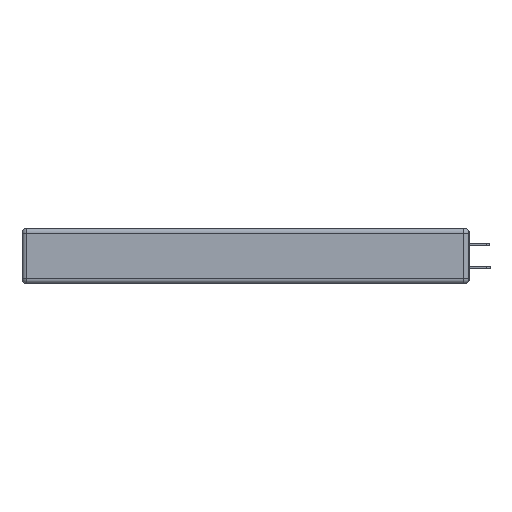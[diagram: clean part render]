
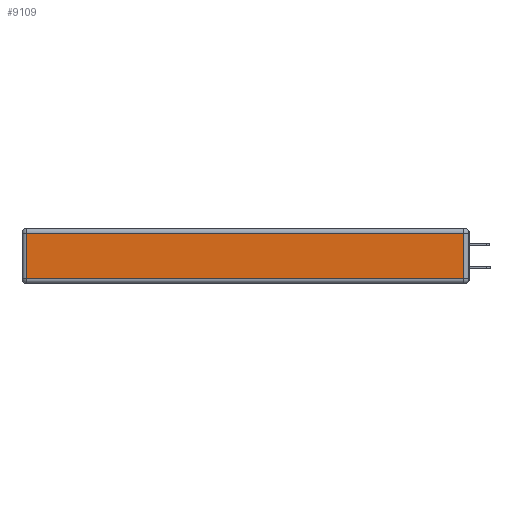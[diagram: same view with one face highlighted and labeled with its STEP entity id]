
A CAD part, left-side view. The second image highlights one B-rep face of the part: STEP entity #9109.
In plain terms, the highlighted planar face has unit normal (-1, 0, 0).
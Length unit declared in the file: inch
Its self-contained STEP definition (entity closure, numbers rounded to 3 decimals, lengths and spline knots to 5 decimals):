
#707 = EDGE_CURVE ( 'NONE', #20774, #18766, #6407, .T. ) ;
#1019 = DIRECTION ( 'NONE',  ( 0., 0., 1. ) ) ;
#1424 = DIRECTION ( 'NONE',  ( 0., 0., -1. ) ) ;
#2869 = EDGE_CURVE ( 'NONE', #13007, #16295, #25251, .T. ) ;
#2914 = VECTOR ( 'NONE', #23460, 39.37008 ) ;
#6209 = CARTESIAN_POINT ( 'NONE',  ( 0., 0.03, -0.03 ) ) ;
#6407 = LINE ( 'NONE', #9385, #2914 ) ;
#7319 = CARTESIAN_POINT ( 'NONE',  ( 0., 2.72, -0.03 ) ) ;
#8759 = CARTESIAN_POINT ( 'NONE',  ( 0., 0.03, -0.343 ) ) ;
#9070 = ORIENTED_EDGE ( 'NONE', *, *, #15851, .T. ) ;
#9109 = ADVANCED_FACE ( 'NONE', ( #24880 ), #24212, .T. ) ;
#9360 = VECTOR ( 'NONE', #1019, 39.37008 ) ;
#9385 = CARTESIAN_POINT ( 'NONE',  ( 0., 0., -0.313 ) ) ;
#9700 = LINE ( 'NONE', #8759, #9360 ) ;
#10495 = DIRECTION ( 'NONE',  ( -1., 0., 0. ) ) ;
#12541 = CARTESIAN_POINT ( 'NONE',  ( 0., 2.72, -0.313 ) ) ;
#13007 = VERTEX_POINT ( 'NONE', #6209 ) ;
#15289 = ORIENTED_EDGE ( 'NONE', *, *, #22993, .T. ) ;
#15851 = EDGE_CURVE ( 'NONE', #16295, #20774, #24227, .T. ) ;
#16295 = VERTEX_POINT ( 'NONE', #7319 ) ;
#16323 = AXIS2_PLACEMENT_3D ( 'NONE', #24485, #10495, #22537 ) ;
#18766 = VERTEX_POINT ( 'NONE', #21510 ) ;
#19129 = CARTESIAN_POINT ( 'NONE',  ( 0., 2.75, -0.03 ) ) ;
#19206 = DIRECTION ( 'NONE',  ( 0., 1., 0. ) ) ;
#19256 = VECTOR ( 'NONE', #19206, 39.37008 ) ;
#19813 = ORIENTED_EDGE ( 'NONE', *, *, #2869, .T. ) ;
#20774 = VERTEX_POINT ( 'NONE', #12541 ) ;
#21510 = CARTESIAN_POINT ( 'NONE',  ( 0., 0.03, -0.313 ) ) ;
#22537 = DIRECTION ( 'NONE',  ( 0., 0., 1. ) ) ;
#22993 = EDGE_CURVE ( 'NONE', #18766, #13007, #9700, .T. ) ;
#23460 = DIRECTION ( 'NONE',  ( 0., -1., 0. ) ) ;
#24212 = PLANE ( 'NONE',  #16323 ) ;
#24227 = LINE ( 'NONE', #25491, #24576 ) ;
#24485 = CARTESIAN_POINT ( 'NONE',  ( 0., 0., -0.343 ) ) ;
#24576 = VECTOR ( 'NONE', #1424, 39.37008 ) ;
#24590 = ORIENTED_EDGE ( 'NONE', *, *, #707, .T. ) ;
#24880 = FACE_OUTER_BOUND ( 'NONE', #25462, .T. ) ;
#25251 = LINE ( 'NONE', #19129, #19256 ) ;
#25462 = EDGE_LOOP ( 'NONE', ( #24590, #15289, #19813, #9070 ) ) ;
#25491 = CARTESIAN_POINT ( 'NONE',  ( 0., 2.72, -0.343 ) ) ;
